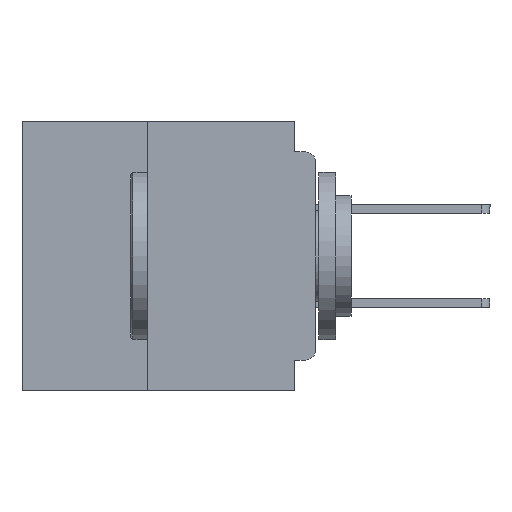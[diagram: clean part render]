
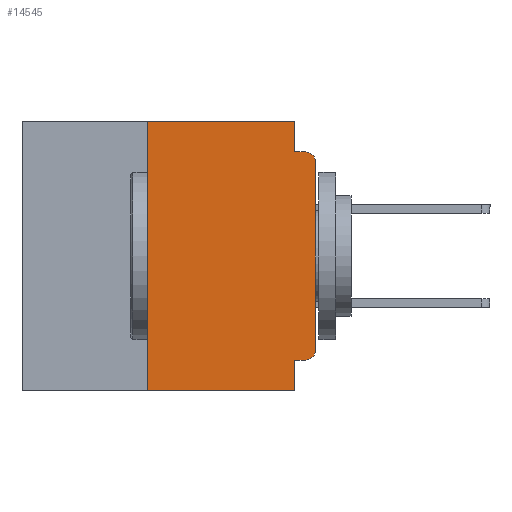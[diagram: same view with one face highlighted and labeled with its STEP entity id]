
A CAD part, left-side view. The second image highlights one B-rep face of the part: STEP entity #14545.
In plain terms, the highlighted planar face has unit normal (-1, 0, 0).
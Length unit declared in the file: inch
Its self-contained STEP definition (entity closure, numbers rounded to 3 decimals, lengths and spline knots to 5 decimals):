
#290 = CARTESIAN_POINT ( 'NONE',  ( 0., 0.015, -0.355 ) ) ;
#393 = CARTESIAN_POINT ( 'NONE',  ( 0., 0.25, -0.4 ) ) ;
#829 = DIRECTION ( 'NONE',  ( -1., 0., 0. ) ) ;
#932 = DIRECTION ( 'NONE',  ( 0., 1., 0. ) ) ;
#1427 = VECTOR ( 'NONE', #36328, 39.37008 ) ;
#1718 = VECTOR ( 'NONE', #14793, 39.37008 ) ;
#1968 = AXIS2_PLACEMENT_3D ( 'NONE', #20012, #829, #23171 ) ;
#3139 = CARTESIAN_POINT ( 'NONE',  ( 0., 0.015, -0.045 ) ) ;
#3609 = DIRECTION ( 'NONE',  ( 0., 0., 1. ) ) ;
#3856 = CIRCLE ( 'NONE', #1968, 0.015 ) ;
#4315 = VERTEX_POINT ( 'NONE', #32972 ) ;
#5034 = CARTESIAN_POINT ( 'NONE',  ( 0., 0.437, 0. ) ) ;
#5416 = AXIS2_PLACEMENT_3D ( 'NONE', #30165, #11152, #33319 ) ;
#6454 = CARTESIAN_POINT ( 'NONE',  ( 0., 0.031, 0. ) ) ;
#6753 = DIRECTION ( 'NONE',  ( 0., 0., -1. ) ) ;
#7335 = VECTOR ( 'NONE', #3609, 39.37008 ) ;
#7616 = CARTESIAN_POINT ( 'NONE',  ( 0., 0.031, -0.045 ) ) ;
#7644 = EDGE_CURVE ( 'NONE', #37356, #35726, #22839, .T. ) ;
#7970 = EDGE_CURVE ( 'NONE', #31230, #4315, #18364, .T. ) ;
#8081 = VERTEX_POINT ( 'NONE', #30170 ) ;
#8894 = CARTESIAN_POINT ( 'NONE',  ( 0., 0., 0. ) ) ;
#9989 = LINE ( 'NONE', #17419, #1427 ) ;
#10375 = ORIENTED_EDGE ( 'NONE', *, *, #7644, .F. ) ;
#10867 = ORIENTED_EDGE ( 'NONE', *, *, #25957, .T. ) ;
#10962 = VERTEX_POINT ( 'NONE', #6454 ) ;
#11152 = DIRECTION ( 'NONE',  ( -1., 0., 0. ) ) ;
#11282 = VECTOR ( 'NONE', #14808, 39.37008 ) ;
#11305 = LINE ( 'NONE', #27366, #1718 ) ;
#12177 = DIRECTION ( 'NONE',  ( 0., 0., 1. ) ) ;
#14545 = ADVANCED_FACE ( 'NONE', ( #29193 ), #33808, .F. ) ;
#14793 = DIRECTION ( 'NONE',  ( 0., -1., 0. ) ) ;
#14808 = DIRECTION ( 'NONE',  ( 0., -1., 0. ) ) ;
#14916 = ORIENTED_EDGE ( 'NONE', *, *, #23173, .F. ) ;
#15270 = CARTESIAN_POINT ( 'NONE',  ( 0., 0.031, -0.355 ) ) ;
#15927 = ORIENTED_EDGE ( 'NONE', *, *, #20886, .T. ) ;
#16018 = EDGE_CURVE ( 'NONE', #10962, #20843, #32498, .T. ) ;
#16975 = VERTEX_POINT ( 'NONE', #33357 ) ;
#17075 = VERTEX_POINT ( 'NONE', #27534 ) ;
#17419 = CARTESIAN_POINT ( 'NONE',  ( 0., 0.437, -0.4 ) ) ;
#17946 = ORIENTED_EDGE ( 'NONE', *, *, #7970, .T. ) ;
#18364 = LINE ( 'NONE', #8894, #35135 ) ;
#20012 = CARTESIAN_POINT ( 'NONE',  ( 0., 0.015, -0.34 ) ) ;
#20163 = EDGE_CURVE ( 'NONE', #35726, #8081, #23975, .T. ) ;
#20843 = VERTEX_POINT ( 'NONE', #7616 ) ;
#20886 = EDGE_CURVE ( 'NONE', #16975, #8081, #9989, .T. ) ;
#21215 = DIRECTION ( 'NONE',  ( 0., 0., -1. ) ) ;
#21994 = VECTOR ( 'NONE', #29786, 39.37008 ) ;
#22355 = VERTEX_POINT ( 'NONE', #3139 ) ;
#22839 = LINE ( 'NONE', #23283, #30285 ) ;
#23171 = DIRECTION ( 'NONE',  ( 0., 0., -1. ) ) ;
#23173 = EDGE_CURVE ( 'NONE', #16975, #17075, #32695, .T. ) ;
#23283 = CARTESIAN_POINT ( 'NONE',  ( 0., 0., -0.355 ) ) ;
#23975 = LINE ( 'NONE', #26561, #21994 ) ;
#25957 = EDGE_CURVE ( 'NONE', #4315, #22355, #29628, .T. ) ;
#26266 = ORIENTED_EDGE ( 'NONE', *, *, #20163, .F. ) ;
#26561 = CARTESIAN_POINT ( 'NONE',  ( 0., 0.031, -0.4 ) ) ;
#27366 = CARTESIAN_POINT ( 'NONE',  ( 0., 0.437, 0. ) ) ;
#27534 = CARTESIAN_POINT ( 'NONE',  ( 0., 0.25, 0. ) ) ;
#27747 = ORIENTED_EDGE ( 'NONE', *, *, #34455, .F. ) ;
#29193 = FACE_OUTER_BOUND ( 'NONE', #39155, .T. ) ;
#29628 = CIRCLE ( 'NONE', #5416, 0.015 ) ;
#29754 = ORIENTED_EDGE ( 'NONE', *, *, #16018, .F. ) ;
#29786 = DIRECTION ( 'NONE',  ( 0., 0., -1. ) ) ;
#30165 = CARTESIAN_POINT ( 'NONE',  ( 0., 0.015, -0.06 ) ) ;
#30170 = CARTESIAN_POINT ( 'NONE',  ( 0., 0.031, -0.4 ) ) ;
#30285 = VECTOR ( 'NONE', #932, 39.37008 ) ;
#31230 = VERTEX_POINT ( 'NONE', #40727 ) ;
#32498 = LINE ( 'NONE', #35341, #40837 ) ;
#32695 = LINE ( 'NONE', #393, #7335 ) ;
#32972 = CARTESIAN_POINT ( 'NONE',  ( 0., 0., -0.06 ) ) ;
#33319 = DIRECTION ( 'NONE',  ( 0., 0., -1. ) ) ;
#33357 = CARTESIAN_POINT ( 'NONE',  ( 0., 0.25, -0.4 ) ) ;
#33730 = CARTESIAN_POINT ( 'NONE',  ( 0., 0., -0.045 ) ) ;
#33808 = PLANE ( 'NONE',  #37174 ) ;
#34455 = EDGE_CURVE ( 'NONE', #20843, #22355, #35534, .T. ) ;
#35135 = VECTOR ( 'NONE', #12177, 39.37008 ) ;
#35341 = CARTESIAN_POINT ( 'NONE',  ( 0., 0.031, 0. ) ) ;
#35534 = LINE ( 'NONE', #33730, #11282 ) ;
#35726 = VERTEX_POINT ( 'NONE', #15270 ) ;
#36328 = DIRECTION ( 'NONE',  ( 0., -1., 0. ) ) ;
#36655 = ORIENTED_EDGE ( 'NONE', *, *, #37454, .T. ) ;
#37174 = AXIS2_PLACEMENT_3D ( 'NONE', #5034, #40095, #21215 ) ;
#37356 = VERTEX_POINT ( 'NONE', #290 ) ;
#37454 = EDGE_CURVE ( 'NONE', #37356, #31230, #3856, .T. ) ;
#38112 = ORIENTED_EDGE ( 'NONE', *, *, #38839, .F. ) ;
#38839 = EDGE_CURVE ( 'NONE', #17075, #10962, #11305, .T. ) ;
#39155 = EDGE_LOOP ( 'NONE', ( #17946, #10867, #27747, #29754, #38112, #14916, #15927, #26266, #10375, #36655 ) ) ;
#40095 = DIRECTION ( 'NONE',  ( 1., 0., 0. ) ) ;
#40727 = CARTESIAN_POINT ( 'NONE',  ( 0., 0., -0.34 ) ) ;
#40837 = VECTOR ( 'NONE', #6753, 39.37008 ) ;
